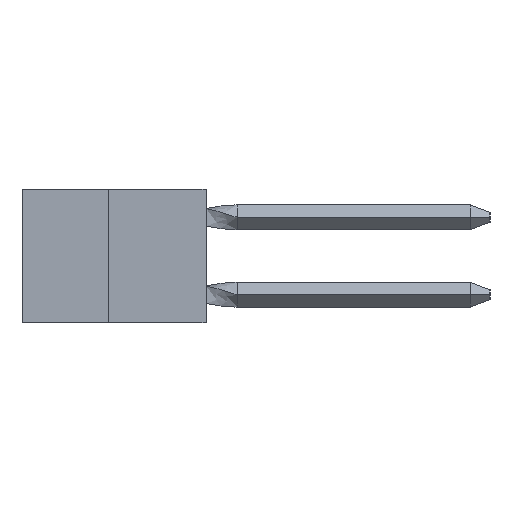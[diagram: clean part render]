
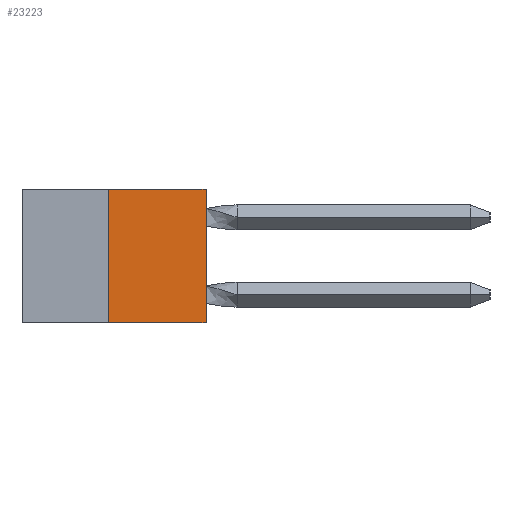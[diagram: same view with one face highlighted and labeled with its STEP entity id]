
A CAD part, left-side view. The second image highlights one B-rep face of the part: STEP entity #23223.
In plain terms, the highlighted planar face has unit normal (-1, 0, 0).
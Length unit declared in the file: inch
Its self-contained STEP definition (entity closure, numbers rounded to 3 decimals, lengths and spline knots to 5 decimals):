
#364 = DIRECTION ( 'NONE',  ( 0., 0., -1. ) ) ;
#3925 = LINE ( 'NONE', #4771, #25466 ) ;
#3977 = ORIENTED_EDGE ( 'NONE', *, *, #12237, .F. ) ;
#4242 = DIRECTION ( 'NONE',  ( 0., 0., 1. ) ) ;
#4658 = VECTOR ( 'NONE', #16186, 39.37008 ) ;
#4771 = CARTESIAN_POINT ( 'NONE',  ( 0., 0., 0. ) ) ;
#8630 = ORIENTED_EDGE ( 'NONE', *, *, #29249, .T. ) ;
#11138 = EDGE_LOOP ( 'NONE', ( #24253, #3977, #26742, #8630 ) ) ;
#11379 = CARTESIAN_POINT ( 'NONE',  ( 0., 0.473, 0. ) ) ;
#11590 = FACE_OUTER_BOUND ( 'NONE', #11138, .T. ) ;
#12237 = EDGE_CURVE ( 'NONE', #32602, #24262, #36223, .T. ) ;
#12840 = DIRECTION ( 'NONE',  ( 0., -1., 0. ) ) ;
#16186 = DIRECTION ( 'NONE',  ( 0., -1., 0. ) ) ;
#16432 = DIRECTION ( 'NONE',  ( 0., 0., 1. ) ) ;
#20636 = LINE ( 'NONE', #31096, #4658 ) ;
#21145 = CARTESIAN_POINT ( 'NONE',  ( 0., 0., -0.343 ) ) ;
#23223 = ADVANCED_FACE ( 'NONE', ( #11590 ), #23316, .F. ) ;
#23316 = PLANE ( 'NONE',  #26657 ) ;
#24253 = ORIENTED_EDGE ( 'NONE', *, *, #31752, .F. ) ;
#24262 = VERTEX_POINT ( 'NONE', #32427 ) ;
#24416 = VERTEX_POINT ( 'NONE', #36213 ) ;
#25466 = VECTOR ( 'NONE', #16432, 39.37008 ) ;
#26657 = AXIS2_PLACEMENT_3D ( 'NONE', #11379, #32308, #364 ) ;
#26742 = ORIENTED_EDGE ( 'NONE', *, *, #38018, .T. ) ;
#28818 = CARTESIAN_POINT ( 'NONE',  ( 0., 0.25, -0.343 ) ) ;
#29249 = EDGE_CURVE ( 'NONE', #37915, #24416, #3925, .T. ) ;
#30721 = LINE ( 'NONE', #33917, #36820 ) ;
#31096 = CARTESIAN_POINT ( 'NONE',  ( 0., 0.473, 0. ) ) ;
#31752 = EDGE_CURVE ( 'NONE', #24262, #24416, #20636, .T. ) ;
#32308 = DIRECTION ( 'NONE',  ( 1., 0., 0. ) ) ;
#32427 = CARTESIAN_POINT ( 'NONE',  ( 0., 0.25, 0. ) ) ;
#32602 = VERTEX_POINT ( 'NONE', #28818 ) ;
#32935 = VECTOR ( 'NONE', #4242, 39.37008 ) ;
#33917 = CARTESIAN_POINT ( 'NONE',  ( 0., 0.473, -0.343 ) ) ;
#36213 = CARTESIAN_POINT ( 'NONE',  ( 0., 0., 0. ) ) ;
#36223 = LINE ( 'NONE', #36712, #32935 ) ;
#36712 = CARTESIAN_POINT ( 'NONE',  ( 0., 0.25, 0. ) ) ;
#36820 = VECTOR ( 'NONE', #12840, 39.37008 ) ;
#37915 = VERTEX_POINT ( 'NONE', #21145 ) ;
#38018 = EDGE_CURVE ( 'NONE', #32602, #37915, #30721, .T. ) ;
